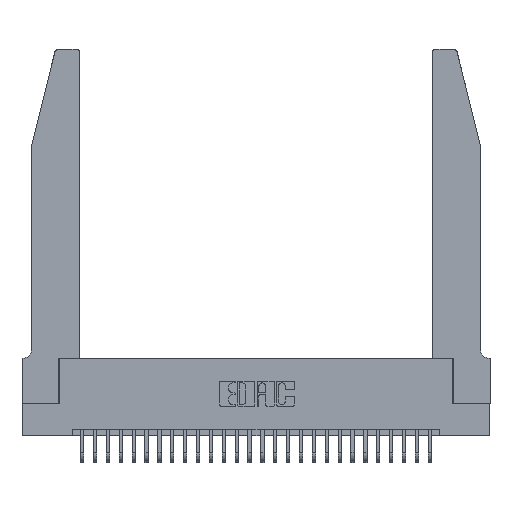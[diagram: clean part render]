
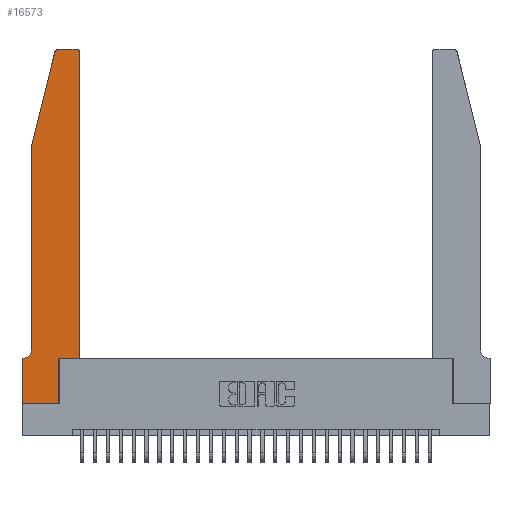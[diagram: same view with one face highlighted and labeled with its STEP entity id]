
A CAD part, top view. The second image highlights one B-rep face of the part: STEP entity #16573.
In plain terms, the highlighted planar face has unit normal (0, 0, 1).
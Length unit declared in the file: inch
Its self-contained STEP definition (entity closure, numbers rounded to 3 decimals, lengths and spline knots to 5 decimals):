
#781 = DIRECTION ( 'NONE',  ( 1., 0., 0. ) ) ;
#1379 = ORIENTED_EDGE ( 'NONE', *, *, #12554, .T. ) ;
#2050 = CIRCLE ( 'NONE', #14298, 0.03 ) ;
#2052 = VERTEX_POINT ( 'NONE', #19378 ) ;
#2121 = VECTOR ( 'NONE', #10820, 39.37008 ) ;
#2202 = EDGE_LOOP ( 'NONE', ( #1379, #2264, #22307, #21200, #14028, #24112, #16598, #20787, #24615, #23139, #5525, #12140 ) ) ;
#2264 = ORIENTED_EDGE ( 'NONE', *, *, #16566, .T. ) ;
#2666 = LINE ( 'NONE', #9213, #26496 ) ;
#2708 = CARTESIAN_POINT ( 'NONE',  ( 0.4205, 2.75, 0.37 ) ) ;
#2720 = CARTESIAN_POINT ( 'NONE',  ( 0.4205, 2.72, 0.37 ) ) ;
#3084 = DIRECTION ( 'NONE',  ( 0., -1., 0. ) ) ;
#3165 = VECTOR ( 'NONE', #6998, 39.37008 ) ;
#3330 = VERTEX_POINT ( 'NONE', #22028 ) ;
#3368 = VERTEX_POINT ( 'NONE', #27524 ) ;
#3386 = CARTESIAN_POINT ( 'NONE',  ( 0.4505, 0.35, 0.37 ) ) ;
#3622 = CARTESIAN_POINT ( 'NONE',  ( 0.0055, 0.42, 0.37 ) ) ;
#3748 = VECTOR ( 'NONE', #22115, 39.37008 ) ;
#3995 = VERTEX_POINT ( 'NONE', #4089 ) ;
#4089 = CARTESIAN_POINT ( 'NONE',  ( 0.25487, 2.72718, 0.37 ) ) ;
#4163 = LINE ( 'NONE', #10234, #21013 ) ;
#5027 = LINE ( 'NONE', #21017, #3165 ) ;
#5328 = CARTESIAN_POINT ( 'NONE',  ( 0.284, 2.72, 0.37 ) ) ;
#5525 = ORIENTED_EDGE ( 'NONE', *, *, #20778, .T. ) ;
#5532 = VECTOR ( 'NONE', #29860, 39.37008 ) ;
#6011 = VERTEX_POINT ( 'NONE', #16680 ) ;
#6364 = DIRECTION ( 'NONE',  ( 0., -1., 0. ) ) ;
#6998 = DIRECTION ( 'NONE',  ( -0.239, -0.971, 0. ) ) ;
#7445 = DIRECTION ( 'NONE',  ( 0., 0., 1. ) ) ;
#7551 = VERTEX_POINT ( 'NONE', #22058 ) ;
#8000 = DIRECTION ( 'NONE',  ( -1., 0., 0. ) ) ;
#8494 = VERTEX_POINT ( 'NONE', #16478 ) ;
#8776 = EDGE_CURVE ( 'NONE', #2052, #12035, #20753, .T. ) ;
#9213 = CARTESIAN_POINT ( 'NONE',  ( 0., 0., 0.37 ) ) ;
#9954 = CARTESIAN_POINT ( 'NONE',  ( 0.2865, 0., 0.37 ) ) ;
#10234 = CARTESIAN_POINT ( 'NONE',  ( 0.0755, 2., 0.37 ) ) ;
#10820 = DIRECTION ( 'NONE',  ( 0., 1., 0. ) ) ;
#11028 = VECTOR ( 'NONE', #27364, 39.37008 ) ;
#11742 = EDGE_CURVE ( 'NONE', #24568, #2052, #24637, .T. ) ;
#11838 = EDGE_CURVE ( 'NONE', #3330, #6011, #22776, .T. ) ;
#12035 = VERTEX_POINT ( 'NONE', #30271 ) ;
#12089 = AXIS2_PLACEMENT_3D ( 'NONE', #3622, #26945, #15198 ) ;
#12140 = ORIENTED_EDGE ( 'NONE', *, *, #14686, .T. ) ;
#12193 = CARTESIAN_POINT ( 'NONE',  ( 0., 0.35, 0.37 ) ) ;
#12387 = PLANE ( 'NONE',  #29536 ) ;
#12554 = EDGE_CURVE ( 'NONE', #25445, #3368, #25313, .T. ) ;
#12617 = CARTESIAN_POINT ( 'NONE',  ( 0.0755, 0.42, 0.37 ) ) ;
#14028 = ORIENTED_EDGE ( 'NONE', *, *, #11742, .T. ) ;
#14298 = AXIS2_PLACEMENT_3D ( 'NONE', #5328, #24129, #781 ) ;
#14686 = EDGE_CURVE ( 'NONE', #8494, #25445, #29958, .T. ) ;
#14719 = DIRECTION ( 'NONE',  ( 1., 0., 0. ) ) ;
#15198 = DIRECTION ( 'NONE',  ( -1., 0., 0. ) ) ;
#16339 = VECTOR ( 'NONE', #8000, 39.37008 ) ;
#16478 = CARTESIAN_POINT ( 'NONE',  ( 0.4505, 2.72, 0.37 ) ) ;
#16566 = EDGE_CURVE ( 'NONE', #3368, #3995, #2050, .T. ) ;
#16573 = ADVANCED_FACE ( 'NONE', ( #21845 ), #12387, .T. ) ;
#16598 = ORIENTED_EDGE ( 'NONE', *, *, #21261, .T. ) ;
#16680 = CARTESIAN_POINT ( 'NONE',  ( 0.4505, 0.35, 0.37 ) ) ;
#17299 = CARTESIAN_POINT ( 'NONE',  ( 0.0755, 0.35, 0.37 ) ) ;
#17533 = LINE ( 'NONE', #29617, #19739 ) ;
#18112 = VERTEX_POINT ( 'NONE', #28140 ) ;
#18338 = EDGE_CURVE ( 'NONE', #7551, #24568, #4163, .T. ) ;
#18842 = EDGE_CURVE ( 'NONE', #18112, #28618, #2666, .T. ) ;
#18981 = DIRECTION ( 'NONE',  ( 1., 0., 0. ) ) ;
#19378 = CARTESIAN_POINT ( 'NONE',  ( 0.0055, 0.35, 0.37 ) ) ;
#19443 = DIRECTION ( 'NONE',  ( 0., 0., 1. ) ) ;
#19739 = VECTOR ( 'NONE', #6364, 39.37008 ) ;
#20409 = CARTESIAN_POINT ( 'NONE',  ( 0.4505, 0.35, 0.37 ) ) ;
#20753 = LINE ( 'NONE', #17299, #16339 ) ;
#20778 = EDGE_CURVE ( 'NONE', #6011, #8494, #20914, .T. ) ;
#20787 = ORIENTED_EDGE ( 'NONE', *, *, #18842, .T. ) ;
#20913 = EDGE_CURVE ( 'NONE', #3995, #7551, #5027, .T. ) ;
#20914 = LINE ( 'NONE', #20409, #5532 ) ;
#21013 = VECTOR ( 'NONE', #3084, 39.37008 ) ;
#21017 = CARTESIAN_POINT ( 'NONE',  ( 0.0755, 2., 0.37 ) ) ;
#21200 = ORIENTED_EDGE ( 'NONE', *, *, #18338, .T. ) ;
#21261 = EDGE_CURVE ( 'NONE', #12035, #18112, #17533, .T. ) ;
#21845 = FACE_OUTER_BOUND ( 'NONE', #2202, .T. ) ;
#22028 = CARTESIAN_POINT ( 'NONE',  ( 0.2865, 0.35, 0.37 ) ) ;
#22058 = CARTESIAN_POINT ( 'NONE',  ( 0.0755, 2., 0.37 ) ) ;
#22115 = DIRECTION ( 'NONE',  ( 1., 0., 0. ) ) ;
#22307 = ORIENTED_EDGE ( 'NONE', *, *, #20913, .T. ) ;
#22776 = LINE ( 'NONE', #3386, #3748 ) ;
#23139 = ORIENTED_EDGE ( 'NONE', *, *, #11838, .T. ) ;
#23876 = AXIS2_PLACEMENT_3D ( 'NONE', #2720, #7445, #28380 ) ;
#24112 = ORIENTED_EDGE ( 'NONE', *, *, #8776, .T. ) ;
#24129 = DIRECTION ( 'NONE',  ( 0., 0., 1. ) ) ;
#24568 = VERTEX_POINT ( 'NONE', #12617 ) ;
#24615 = ORIENTED_EDGE ( 'NONE', *, *, #26473, .T. ) ;
#24637 = CIRCLE ( 'NONE', #12089, 0.07 ) ;
#25255 = LINE ( 'NONE', #27458, #2121 ) ;
#25313 = LINE ( 'NONE', #26972, #11028 ) ;
#25445 = VERTEX_POINT ( 'NONE', #2708 ) ;
#26473 = EDGE_CURVE ( 'NONE', #28618, #3330, #25255, .T. ) ;
#26496 = VECTOR ( 'NONE', #18981, 39.37008 ) ;
#26945 = DIRECTION ( 'NONE',  ( 0., 0., -1. ) ) ;
#26972 = CARTESIAN_POINT ( 'NONE',  ( 0.2605, 2.75, 0.37 ) ) ;
#27364 = DIRECTION ( 'NONE',  ( -1., 0., 0. ) ) ;
#27458 = CARTESIAN_POINT ( 'NONE',  ( 0.2865, 0.35, 0.37 ) ) ;
#27524 = CARTESIAN_POINT ( 'NONE',  ( 0.284, 2.75, 0.37 ) ) ;
#28140 = CARTESIAN_POINT ( 'NONE',  ( 0., 0., 0.37 ) ) ;
#28380 = DIRECTION ( 'NONE',  ( 1., 0., 0. ) ) ;
#28618 = VERTEX_POINT ( 'NONE', #9954 ) ;
#29536 = AXIS2_PLACEMENT_3D ( 'NONE', #12193, #19443, #14719 ) ;
#29617 = CARTESIAN_POINT ( 'NONE',  ( 0., 0., 0.37 ) ) ;
#29860 = DIRECTION ( 'NONE',  ( 0., 1., 0. ) ) ;
#29958 = CIRCLE ( 'NONE', #23876, 0.03 ) ;
#30271 = CARTESIAN_POINT ( 'NONE',  ( 0., 0.35, 0.37 ) ) ;
